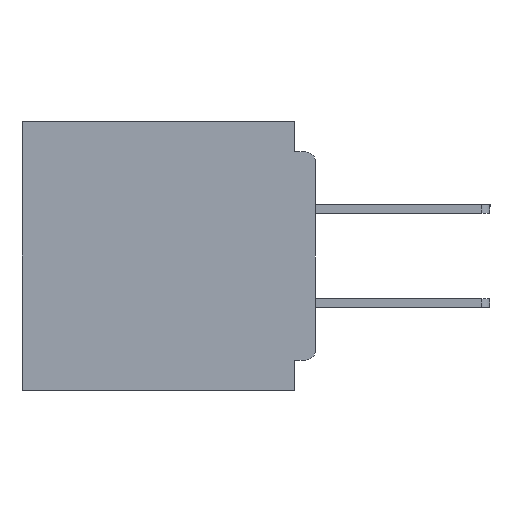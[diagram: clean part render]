
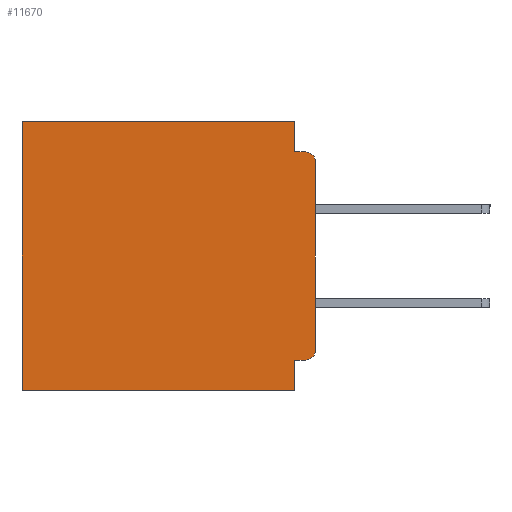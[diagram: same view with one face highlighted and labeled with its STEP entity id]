
A CAD part, left-side view. The second image highlights one B-rep face of the part: STEP entity #11670.
In plain terms, the highlighted planar face has unit normal (-1, 0, 0).
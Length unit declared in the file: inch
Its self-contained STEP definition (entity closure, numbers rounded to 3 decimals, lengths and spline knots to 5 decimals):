
#15 = CARTESIAN_POINT ( 'NONE',  ( 0.3, 0., 0. ) ) ;
#220 = VERTEX_POINT ( 'NONE', #54438 ) ;
#386 = ORIENTED_EDGE ( 'NONE', *, *, #48109, .T. ) ;
#1040 = ORIENTED_EDGE ( 'NONE', *, *, #17039, .T. ) ;
#1532 = CARTESIAN_POINT ( 'NONE',  ( 0.3, 0., -0.06 ) ) ;
#3511 = ORIENTED_EDGE ( 'NONE', *, *, #38492, .F. ) ;
#4816 = VERTEX_POINT ( 'NONE', #31589 ) ;
#5070 = DIRECTION ( 'NONE',  ( 1., 0., 0. ) ) ;
#5600 = VECTOR ( 'NONE', #26067, 39.37008 ) ;
#6759 = ORIENTED_EDGE ( 'NONE', *, *, #21106, .T. ) ;
#6907 = FACE_OUTER_BOUND ( 'NONE', #20449, .T. ) ;
#7139 = ORIENTED_EDGE ( 'NONE', *, *, #28190, .F. ) ;
#7987 = CARTESIAN_POINT ( 'NONE',  ( 0.3, 0., -0.355 ) ) ;
#10905 = LINE ( 'NONE', #59644, #35405 ) ;
#11097 = LINE ( 'NONE', #15, #60076 ) ;
#11670 = ADVANCED_FACE ( 'NONE', ( #6907 ), #29429, .F. ) ;
#12821 = CARTESIAN_POINT ( 'NONE',  ( 0.3, 0., -0.045 ) ) ;
#14866 = DIRECTION ( 'NONE',  ( 0., 1., 0. ) ) ;
#17039 = EDGE_CURVE ( 'NONE', #34027, #220, #48111, .T. ) ;
#18191 = CARTESIAN_POINT ( 'NONE',  ( 0.3, 0.015, -0.34 ) ) ;
#18845 = DIRECTION ( 'NONE',  ( -1., 0., 0. ) ) ;
#19194 = LINE ( 'NONE', #61039, #42218 ) ;
#19580 = CARTESIAN_POINT ( 'NONE',  ( 0.3, 0., -0.4 ) ) ;
#20449 = EDGE_LOOP ( 'NONE', ( #35143, #386, #7139, #36046, #6759, #1040, #37064, #58482, #3511, #21121 ) ) ;
#21106 = EDGE_CURVE ( 'NONE', #37437, #34027, #11097, .T. ) ;
#21121 = ORIENTED_EDGE ( 'NONE', *, *, #23422, .T. ) ;
#22455 = EDGE_CURVE ( 'NONE', #33250, #34275, #10905, .T. ) ;
#22891 = DIRECTION ( 'NONE',  ( 0., 0., -1. ) ) ;
#23108 = DIRECTION ( 'NONE',  ( 0., 0., -1. ) ) ;
#23277 = CARTESIAN_POINT ( 'NONE',  ( 0.3, 0.015, -0.045 ) ) ;
#23422 = EDGE_CURVE ( 'NONE', #50616, #34275, #42165, .T. ) ;
#23960 = AXIS2_PLACEMENT_3D ( 'NONE', #19580, #5070, #39346 ) ;
#26067 = DIRECTION ( 'NONE',  ( 0., 0., -1. ) ) ;
#26728 = DIRECTION ( 'NONE',  ( 0., 0., -1. ) ) ;
#26954 = VECTOR ( 'NONE', #61816, 39.37008 ) ;
#27430 = EDGE_CURVE ( 'NONE', #37437, #62788, #43118, .T. ) ;
#27645 = CARTESIAN_POINT ( 'NONE',  ( 0.3, 0.031, -0.045 ) ) ;
#28190 = EDGE_CURVE ( 'NONE', #62788, #31018, #40077, .T. ) ;
#29429 = PLANE ( 'NONE',  #23960 ) ;
#30078 = CARTESIAN_POINT ( 'NONE',  ( 0.3, 0.031, 0. ) ) ;
#31018 = VERTEX_POINT ( 'NONE', #23277 ) ;
#31589 = CARTESIAN_POINT ( 'NONE',  ( 0.3, 0.031, -0.355 ) ) ;
#33246 = VERTEX_POINT ( 'NONE', #60198 ) ;
#33250 = VERTEX_POINT ( 'NONE', #1532 ) ;
#33291 = AXIS2_PLACEMENT_3D ( 'NONE', #18191, #52500, #23108 ) ;
#33386 = EDGE_CURVE ( 'NONE', #4816, #33246, #19194, .T. ) ;
#33550 = VECTOR ( 'NONE', #22891, 39.37008 ) ;
#34027 = VERTEX_POINT ( 'NONE', #56076 ) ;
#34275 = VERTEX_POINT ( 'NONE', #48514 ) ;
#35143 = ORIENTED_EDGE ( 'NONE', *, *, #22455, .F. ) ;
#35388 = LINE ( 'NONE', #7987, #59869 ) ;
#35405 = VECTOR ( 'NONE', #49806, 39.37008 ) ;
#36046 = ORIENTED_EDGE ( 'NONE', *, *, #27430, .F. ) ;
#36647 = DIRECTION ( 'NONE',  ( 0., 1., 0. ) ) ;
#37064 = ORIENTED_EDGE ( 'NONE', *, *, #57388, .F. ) ;
#37437 = VERTEX_POINT ( 'NONE', #30078 ) ;
#38492 = EDGE_CURVE ( 'NONE', #50616, #4816, #35388, .T. ) ;
#39346 = DIRECTION ( 'NONE',  ( 0., 0., -1. ) ) ;
#40077 = LINE ( 'NONE', #12821, #26954 ) ;
#41329 = AXIS2_PLACEMENT_3D ( 'NONE', #48210, #18845, #53164 ) ;
#42165 = CIRCLE ( 'NONE', #33291, 0.015 ) ;
#42211 = DIRECTION ( 'NONE',  ( 0., 1., 0. ) ) ;
#42218 = VECTOR ( 'NONE', #26728, 39.37008 ) ;
#43118 = LINE ( 'NONE', #45594, #5600 ) ;
#45594 = CARTESIAN_POINT ( 'NONE',  ( 0.3, 0.031, 0. ) ) ;
#47314 = CARTESIAN_POINT ( 'NONE',  ( 0.3, 0.437, -0.4 ) ) ;
#48109 = EDGE_CURVE ( 'NONE', #33250, #31018, #62589, .T. ) ;
#48111 = LINE ( 'NONE', #47314, #33550 ) ;
#48210 = CARTESIAN_POINT ( 'NONE',  ( 0.3, 0.015, -0.06 ) ) ;
#48514 = CARTESIAN_POINT ( 'NONE',  ( 0.3, 0., -0.34 ) ) ;
#49806 = DIRECTION ( 'NONE',  ( 0., 0., -1. ) ) ;
#49914 = VECTOR ( 'NONE', #36647, 39.37008 ) ;
#50616 = VERTEX_POINT ( 'NONE', #52626 ) ;
#52500 = DIRECTION ( 'NONE',  ( -1., 0., 0. ) ) ;
#52626 = CARTESIAN_POINT ( 'NONE',  ( 0.3, 0.015, -0.355 ) ) ;
#53164 = DIRECTION ( 'NONE',  ( 0., 0., -1. ) ) ;
#54438 = CARTESIAN_POINT ( 'NONE',  ( 0.3, 0.437, -0.4 ) ) ;
#56076 = CARTESIAN_POINT ( 'NONE',  ( 0.3, 0.437, 0. ) ) ;
#56137 = CARTESIAN_POINT ( 'NONE',  ( 0.3, 0., -0.4 ) ) ;
#57388 = EDGE_CURVE ( 'NONE', #33246, #220, #62943, .T. ) ;
#58482 = ORIENTED_EDGE ( 'NONE', *, *, #33386, .F. ) ;
#59644 = CARTESIAN_POINT ( 'NONE',  ( 0.3, 0., -0.4 ) ) ;
#59869 = VECTOR ( 'NONE', #42211, 39.37008 ) ;
#60076 = VECTOR ( 'NONE', #14866, 39.37008 ) ;
#60198 = CARTESIAN_POINT ( 'NONE',  ( 0.3, 0.031, -0.4 ) ) ;
#61039 = CARTESIAN_POINT ( 'NONE',  ( 0.3, 0.031, -0.4 ) ) ;
#61816 = DIRECTION ( 'NONE',  ( 0., -1., 0. ) ) ;
#62589 = CIRCLE ( 'NONE', #41329, 0.015 ) ;
#62788 = VERTEX_POINT ( 'NONE', #27645 ) ;
#62943 = LINE ( 'NONE', #56137, #49914 ) ;
